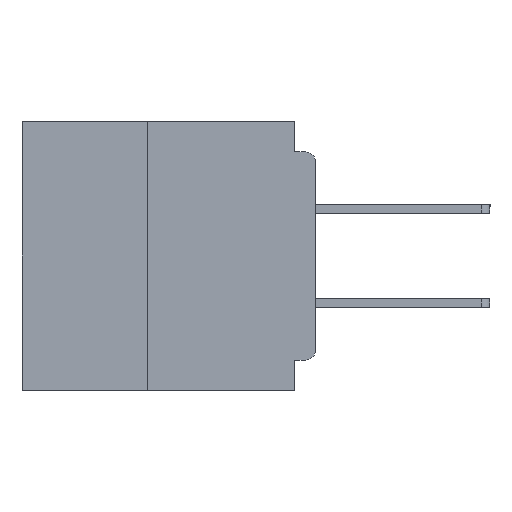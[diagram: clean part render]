
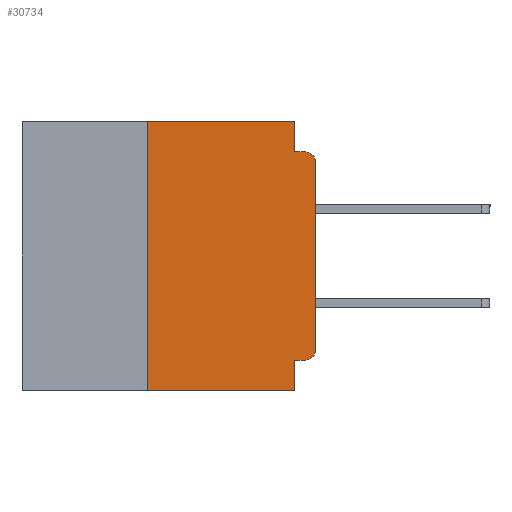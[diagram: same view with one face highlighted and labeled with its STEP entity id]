
A CAD part, left-side view. The second image highlights one B-rep face of the part: STEP entity #30734.
In plain terms, the highlighted planar face has unit normal (-1, 0, 0).
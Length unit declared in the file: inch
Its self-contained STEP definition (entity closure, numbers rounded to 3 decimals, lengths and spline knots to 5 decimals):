
#573 = EDGE_CURVE ( 'NONE', #13582, #23336, #26761, .T. ) ;
#834 = AXIS2_PLACEMENT_3D ( 'NONE', #33199, #16191, #35933 ) ;
#1312 = LINE ( 'NONE', #16130, #23328 ) ;
#1755 = VERTEX_POINT ( 'NONE', #30430 ) ;
#1838 = EDGE_CURVE ( 'NONE', #9169, #21921, #35845, .T. ) ;
#2825 = EDGE_CURVE ( 'NONE', #15465, #8598, #3754, .T. ) ;
#2891 = CARTESIAN_POINT ( 'NONE',  ( 0., 0., -0.34 ) ) ;
#3057 = ORIENTED_EDGE ( 'NONE', *, *, #6708, .F. ) ;
#3083 = ORIENTED_EDGE ( 'NONE', *, *, #19266, .F. ) ;
#3115 = DIRECTION ( 'NONE',  ( 0., 0., -1. ) ) ;
#3754 = LINE ( 'NONE', #36197, #10439 ) ;
#4211 = VERTEX_POINT ( 'NONE', #27258 ) ;
#4541 = LINE ( 'NONE', #20333, #33126 ) ;
#4904 = VECTOR ( 'NONE', #7367, 39.37008 ) ;
#6177 = DIRECTION ( 'NONE',  ( 0., 0., 1. ) ) ;
#6478 = CIRCLE ( 'NONE', #834, 0.015 ) ;
#6708 = EDGE_CURVE ( 'NONE', #4211, #13582, #1312, .T. ) ;
#7367 = DIRECTION ( 'NONE',  ( 0., -1., 0. ) ) ;
#8019 = CARTESIAN_POINT ( 'NONE',  ( 0., 0., -0.06 ) ) ;
#8598 = VERTEX_POINT ( 'NONE', #8019 ) ;
#8807 = EDGE_CURVE ( 'NONE', #30220, #9169, #34171, .T. ) ;
#8968 = AXIS2_PLACEMENT_3D ( 'NONE', #27222, #10033, #30101 ) ;
#9169 = VERTEX_POINT ( 'NONE', #22217 ) ;
#9979 = VECTOR ( 'NONE', #17769, 39.37008 ) ;
#10033 = DIRECTION ( 'NONE',  ( -1., 0., 0. ) ) ;
#10252 = EDGE_CURVE ( 'NONE', #4211, #15465, #26778, .T. ) ;
#10439 = VECTOR ( 'NONE', #18225, 39.37008 ) ;
#11260 = CARTESIAN_POINT ( 'NONE',  ( 0., 0.437, 0. ) ) ;
#11602 = ORIENTED_EDGE ( 'NONE', *, *, #573, .F. ) ;
#12002 = ORIENTED_EDGE ( 'NONE', *, *, #13439, .T. ) ;
#12328 = VECTOR ( 'NONE', #6177, 39.37008 ) ;
#12521 = CARTESIAN_POINT ( 'NONE',  ( 0., 0.031, -0.355 ) ) ;
#12790 = DIRECTION ( 'NONE',  ( 0., 0., -1. ) ) ;
#13439 = EDGE_CURVE ( 'NONE', #30220, #23336, #26151, .T. ) ;
#13582 = VERTEX_POINT ( 'NONE', #12521 ) ;
#13659 = ORIENTED_EDGE ( 'NONE', *, *, #8807, .F. ) ;
#13974 = CARTESIAN_POINT ( 'NONE',  ( 0., 0.437, 0. ) ) ;
#14114 = ORIENTED_EDGE ( 'NONE', *, *, #1838, .F. ) ;
#14477 = DIRECTION ( 'NONE',  ( 0., -1., 0. ) ) ;
#14571 = EDGE_CURVE ( 'NONE', #21921, #23857, #4541, .T. ) ;
#15179 = CARTESIAN_POINT ( 'NONE',  ( 0., 0.031, -0.045 ) ) ;
#15465 = VERTEX_POINT ( 'NONE', #2891 ) ;
#15567 = CARTESIAN_POINT ( 'NONE',  ( 0., 0.031, 0. ) ) ;
#16081 = CARTESIAN_POINT ( 'NONE',  ( 0., 0., -0.045 ) ) ;
#16130 = CARTESIAN_POINT ( 'NONE',  ( 0., 0., -0.355 ) ) ;
#16191 = DIRECTION ( 'NONE',  ( -1., 0., 0. ) ) ;
#16977 = PLANE ( 'NONE',  #26776 ) ;
#17270 = ORIENTED_EDGE ( 'NONE', *, *, #29375, .T. ) ;
#17456 = ORIENTED_EDGE ( 'NONE', *, *, #2825, .T. ) ;
#17769 = DIRECTION ( 'NONE',  ( 0., -1., 0. ) ) ;
#18225 = DIRECTION ( 'NONE',  ( 0., 0., 1. ) ) ;
#19266 = EDGE_CURVE ( 'NONE', #23857, #1755, #35197, .T. ) ;
#20010 = DIRECTION ( 'NONE',  ( 0., 0., -1. ) ) ;
#20333 = CARTESIAN_POINT ( 'NONE',  ( 0., 0.031, 0. ) ) ;
#20650 = CARTESIAN_POINT ( 'NONE',  ( 0., 0.437, -0.4 ) ) ;
#21628 = CARTESIAN_POINT ( 'NONE',  ( 0., 0.031, -0.4 ) ) ;
#21921 = VERTEX_POINT ( 'NONE', #15567 ) ;
#22217 = CARTESIAN_POINT ( 'NONE',  ( 0., 0.25, 0. ) ) ;
#23139 = ORIENTED_EDGE ( 'NONE', *, *, #14571, .F. ) ;
#23328 = VECTOR ( 'NONE', #27621, 39.37008 ) ;
#23336 = VERTEX_POINT ( 'NONE', #21628 ) ;
#23857 = VERTEX_POINT ( 'NONE', #15179 ) ;
#25625 = CARTESIAN_POINT ( 'NONE',  ( 0., 0.25, -0.4 ) ) ;
#25897 = VECTOR ( 'NONE', #12790, 39.37008 ) ;
#26151 = LINE ( 'NONE', #20650, #9979 ) ;
#26208 = CARTESIAN_POINT ( 'NONE',  ( 0., 0.25, -0.4 ) ) ;
#26761 = LINE ( 'NONE', #33206, #25897 ) ;
#26776 = AXIS2_PLACEMENT_3D ( 'NONE', #11260, #36774, #20010 ) ;
#26778 = CIRCLE ( 'NONE', #8968, 0.015 ) ;
#27222 = CARTESIAN_POINT ( 'NONE',  ( 0., 0.015, -0.34 ) ) ;
#27258 = CARTESIAN_POINT ( 'NONE',  ( 0., 0.015, -0.355 ) ) ;
#27438 = FACE_OUTER_BOUND ( 'NONE', #31998, .T. ) ;
#27621 = DIRECTION ( 'NONE',  ( 0., 1., 0. ) ) ;
#28483 = VECTOR ( 'NONE', #14477, 39.37008 ) ;
#29375 = EDGE_CURVE ( 'NONE', #8598, #1755, #6478, .T. ) ;
#30101 = DIRECTION ( 'NONE',  ( 0., 0., -1. ) ) ;
#30220 = VERTEX_POINT ( 'NONE', #25625 ) ;
#30430 = CARTESIAN_POINT ( 'NONE',  ( 0., 0.015, -0.045 ) ) ;
#30734 = ADVANCED_FACE ( 'NONE', ( #27438 ), #16977, .F. ) ;
#31998 = EDGE_LOOP ( 'NONE', ( #17456, #17270, #3083, #23139, #14114, #13659, #12002, #11602, #3057, #32843 ) ) ;
#32843 = ORIENTED_EDGE ( 'NONE', *, *, #10252, .T. ) ;
#33126 = VECTOR ( 'NONE', #3115, 39.37008 ) ;
#33199 = CARTESIAN_POINT ( 'NONE',  ( 0., 0.015, -0.06 ) ) ;
#33206 = CARTESIAN_POINT ( 'NONE',  ( 0., 0.031, -0.4 ) ) ;
#34171 = LINE ( 'NONE', #26208, #12328 ) ;
#35197 = LINE ( 'NONE', #16081, #4904 ) ;
#35845 = LINE ( 'NONE', #13974, #28483 ) ;
#35933 = DIRECTION ( 'NONE',  ( 0., 0., -1. ) ) ;
#36197 = CARTESIAN_POINT ( 'NONE',  ( 0., 0., 0. ) ) ;
#36774 = DIRECTION ( 'NONE',  ( 1., 0., 0. ) ) ;
